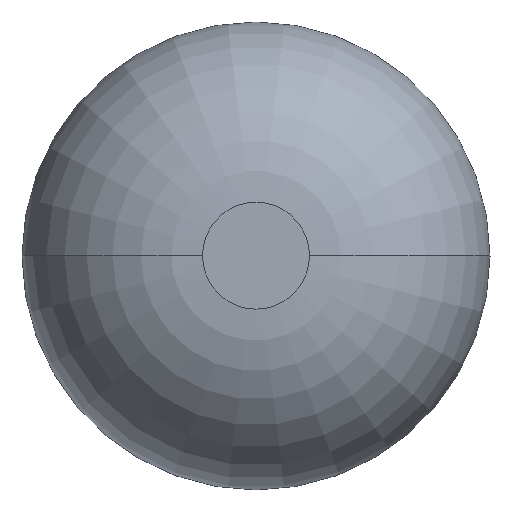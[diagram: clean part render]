
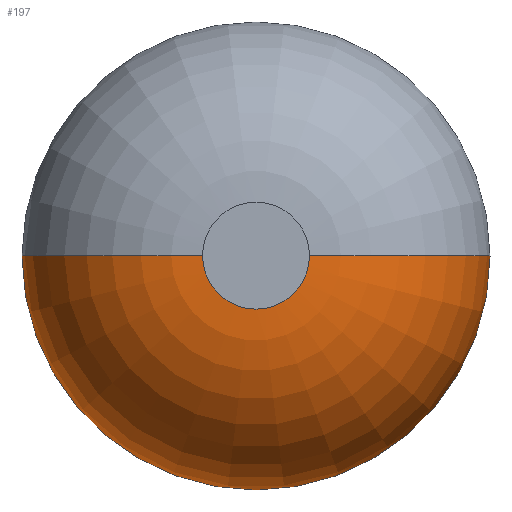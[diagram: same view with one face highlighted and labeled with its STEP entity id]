
A CAD part, top view. The second image highlights one B-rep face of the part: STEP entity #197.
In plain terms, the highlighted toroidal (fillet/blend) face has major radius 7.523 mm and minor radius 25.4 mm.
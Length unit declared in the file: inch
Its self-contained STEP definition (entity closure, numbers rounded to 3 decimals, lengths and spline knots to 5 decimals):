
#8 = DIRECTION ( 'NONE',  ( 0., 0., 1. ) ) ;
#12 = EDGE_LOOP ( 'NONE', ( #77, #126, #133, #150 ) ) ;
#14 = CIRCLE ( 'NONE', #167, 1. ) ;
#26 = CIRCLE ( 'NONE', #128, 1. ) ;
#27 = EDGE_CURVE ( 'NONE', #87, #36, #14, .T. ) ;
#36 = VERTEX_POINT ( 'NONE', #238 ) ;
#37 = EDGE_CURVE ( 'NONE', #242, #200, #26, .T. ) ;
#41 = EDGE_CURVE ( 'NONE', #87, #242, #262, .T. ) ;
#56 = CIRCLE ( 'NONE', #226, 0.29618 ) ;
#61 = CARTESIAN_POINT ( 'NONE',  ( 43.1249, 13.36331, 3. ) ) ;
#77 = ORIENTED_EDGE ( 'NONE', *, *, #27, .F. ) ;
#87 = VERTEX_POINT ( 'NONE', #61 ) ;
#98 = DIRECTION ( 'NONE',  ( 1., 0., 0. ) ) ;
#117 = DIRECTION ( 'NONE',  ( 0., 0., 1. ) ) ;
#118 = CARTESIAN_POINT ( 'NONE',  ( 44.42108, 13.36331, 3. ) ) ;
#124 = DIRECTION ( 'NONE',  ( 0., 0., -1. ) ) ;
#126 = ORIENTED_EDGE ( 'NONE', *, *, #41, .T. ) ;
#128 = AXIS2_PLACEMENT_3D ( 'NONE', #145, #142, #124 ) ;
#129 = TOROIDAL_SURFACE ( 'NONE', #235, 0.29618, 1. ) ;
#133 = ORIENTED_EDGE ( 'NONE', *, *, #37, .T. ) ;
#142 = DIRECTION ( 'NONE',  ( 0., -1., 0. ) ) ;
#145 = CARTESIAN_POINT ( 'NONE',  ( 44.71726, 13.36331, 3. ) ) ;
#150 = ORIENTED_EDGE ( 'NONE', *, *, #218, .F. ) ;
#167 = AXIS2_PLACEMENT_3D ( 'NONE', #181, #179, #177 ) ;
#177 = DIRECTION ( 'NONE',  ( -1., 0., 0. ) ) ;
#179 = DIRECTION ( 'NONE',  ( 0., 1., 0. ) ) ;
#181 = CARTESIAN_POINT ( 'NONE',  ( 44.1249, 13.36331, 3. ) ) ;
#197 = ADVANCED_FACE ( 'NONE', ( #232 ), #129, .T. ) ;
#200 = VERTEX_POINT ( 'NONE', #277 ) ;
#205 = AXIS2_PLACEMENT_3D ( 'NONE', #118, #117, #98 ) ;
#218 = EDGE_CURVE ( 'NONE', #36, #200, #56, .T. ) ;
#220 = DIRECTION ( 'NONE',  ( 1., 0., 0. ) ) ;
#223 = DIRECTION ( 'NONE',  ( 0., 0., 1. ) ) ;
#225 = CARTESIAN_POINT ( 'NONE',  ( 44.42108, 13.36331, 4. ) ) ;
#226 = AXIS2_PLACEMENT_3D ( 'NONE', #225, #223, #220 ) ;
#232 = FACE_OUTER_BOUND ( 'NONE', #12, .T. ) ;
#235 = AXIS2_PLACEMENT_3D ( 'NONE', #282, #8, #278 ) ;
#238 = CARTESIAN_POINT ( 'NONE',  ( 44.1249, 13.36331, 4. ) ) ;
#242 = VERTEX_POINT ( 'NONE', #245 ) ;
#245 = CARTESIAN_POINT ( 'NONE',  ( 45.71726, 13.36331, 3. ) ) ;
#262 = CIRCLE ( 'NONE', #205, 1.29618 ) ;
#277 = CARTESIAN_POINT ( 'NONE',  ( 44.71726, 13.36331, 4. ) ) ;
#278 = DIRECTION ( 'NONE',  ( 1., 0., 0. ) ) ;
#282 = CARTESIAN_POINT ( 'NONE',  ( 44.42108, 13.36331, 3. ) ) ;
